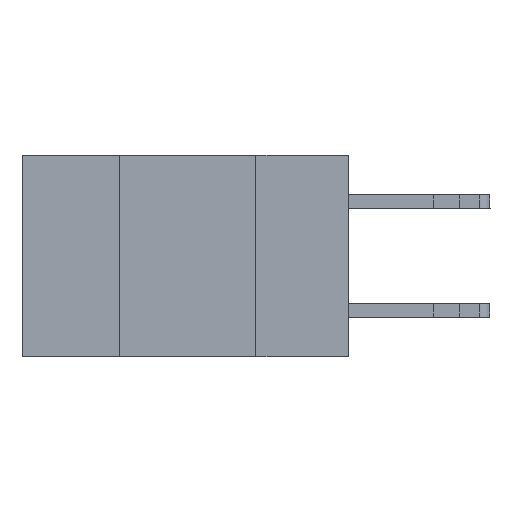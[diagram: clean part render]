
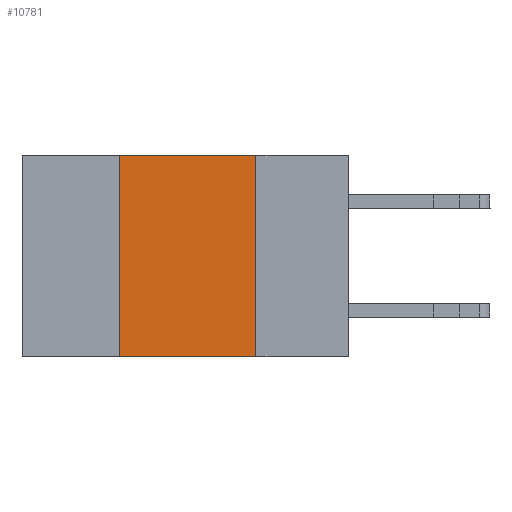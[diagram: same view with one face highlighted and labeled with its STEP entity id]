
A CAD part, left-side view. The second image highlights one B-rep face of the part: STEP entity #10781.
In plain terms, the highlighted planar face has unit normal (-1, 0, 0).
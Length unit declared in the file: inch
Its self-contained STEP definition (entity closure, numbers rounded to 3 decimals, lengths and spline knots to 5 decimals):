
#318 = ORIENTED_EDGE ( 'NONE', *, *, #2191, .T. ) ;
#747 = PLANE ( 'NONE',  #4493 ) ;
#750 = CARTESIAN_POINT ( 'NONE',  ( 0., 0.17, -0.37 ) ) ;
#1362 = VERTEX_POINT ( 'NONE', #6884 ) ;
#1447 = CARTESIAN_POINT ( 'NONE',  ( 0., 0.17, 0. ) ) ;
#1453 = VERTEX_POINT ( 'NONE', #4645 ) ;
#1806 = LINE ( 'NONE', #3716, #4286 ) ;
#1826 = VERTEX_POINT ( 'NONE', #750 ) ;
#2191 = EDGE_CURVE ( 'NONE', #1453, #1826, #10057, .T. ) ;
#2343 = LINE ( 'NONE', #1447, #7385 ) ;
#2720 = DIRECTION ( 'NONE',  ( 0., 0., -1. ) ) ;
#3223 = CARTESIAN_POINT ( 'NONE',  ( 0., 0.6, -0.37 ) ) ;
#3521 = ORIENTED_EDGE ( 'NONE', *, *, #7279, .F. ) ;
#3666 = ORIENTED_EDGE ( 'NONE', *, *, #9904, .F. ) ;
#3716 = CARTESIAN_POINT ( 'NONE',  ( 0., 0.6, 0. ) ) ;
#4286 = VECTOR ( 'NONE', #7580, 39.37008 ) ;
#4493 = AXIS2_PLACEMENT_3D ( 'NONE', #5439, #8552, #2720 ) ;
#4645 = CARTESIAN_POINT ( 'NONE',  ( 0., 0.42, -0.37 ) ) ;
#5154 = VECTOR ( 'NONE', #7749, 39.37008 ) ;
#5299 = DIRECTION ( 'NONE',  ( 0., 0., -1. ) ) ;
#5439 = CARTESIAN_POINT ( 'NONE',  ( 0., 0.6, 0. ) ) ;
#6294 = ORIENTED_EDGE ( 'NONE', *, *, #7582, .F. ) ;
#6518 = FACE_OUTER_BOUND ( 'NONE', #10177, .T. ) ;
#6884 = CARTESIAN_POINT ( 'NONE',  ( 0., 0.17, 0. ) ) ;
#7279 = EDGE_CURVE ( 'NONE', #1453, #10967, #9633, .T. ) ;
#7385 = VECTOR ( 'NONE', #5299, 39.37008 ) ;
#7580 = DIRECTION ( 'NONE',  ( 0., -1., 0. ) ) ;
#7582 = EDGE_CURVE ( 'NONE', #1362, #1826, #2343, .T. ) ;
#7625 = CARTESIAN_POINT ( 'NONE',  ( 0., 0.42, 0. ) ) ;
#7749 = DIRECTION ( 'NONE',  ( 0., 0., 1. ) ) ;
#7757 = VECTOR ( 'NONE', #9158, 39.37008 ) ;
#8552 = DIRECTION ( 'NONE',  ( 1., 0., 0. ) ) ;
#9158 = DIRECTION ( 'NONE',  ( 0., -1., 0. ) ) ;
#9633 = LINE ( 'NONE', #7625, #5154 ) ;
#9904 = EDGE_CURVE ( 'NONE', #10967, #1362, #1806, .T. ) ;
#10057 = LINE ( 'NONE', #3223, #7757 ) ;
#10177 = EDGE_LOOP ( 'NONE', ( #6294, #3666, #3521, #318 ) ) ;
#10564 = CARTESIAN_POINT ( 'NONE',  ( 0., 0.42, 0. ) ) ;
#10781 = ADVANCED_FACE ( 'NONE', ( #6518 ), #747, .F. ) ;
#10967 = VERTEX_POINT ( 'NONE', #10564 ) ;
